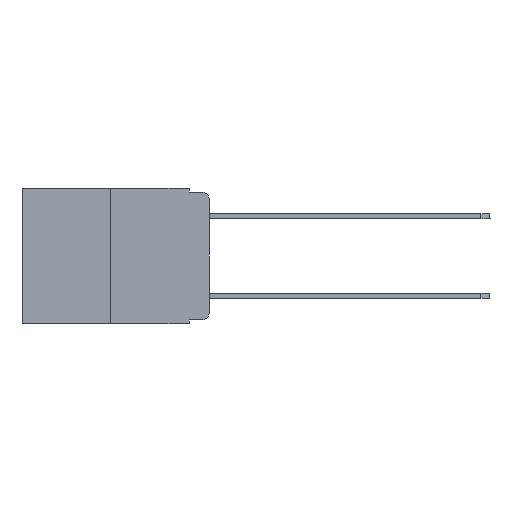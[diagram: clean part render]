
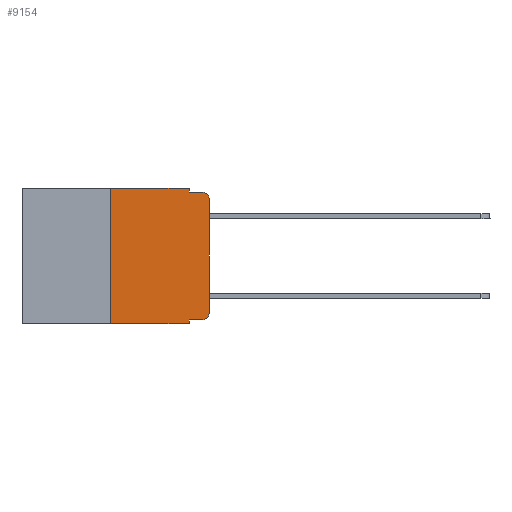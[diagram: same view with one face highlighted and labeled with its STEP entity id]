
A CAD part, left-side view. The second image highlights one B-rep face of the part: STEP entity #9154.
In plain terms, the highlighted planar face has unit normal (-1, 0, 0).
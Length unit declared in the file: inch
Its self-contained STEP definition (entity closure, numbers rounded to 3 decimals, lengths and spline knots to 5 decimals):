
#25 = VERTEX_POINT ( 'NONE', #19356 ) ;
#434 = LINE ( 'NONE', #15198, #15115 ) ;
#866 = EDGE_CURVE ( 'NONE', #24157, #17424, #7147, .T. ) ;
#1061 = VERTEX_POINT ( 'NONE', #18509 ) ;
#1242 = CARTESIAN_POINT ( 'NONE',  ( 0., 0.02, -0.01 ) ) ;
#1291 = VERTEX_POINT ( 'NONE', #17629 ) ;
#1494 = VECTOR ( 'NONE', #23432, 39.37008 ) ;
#1907 = CARTESIAN_POINT ( 'NONE',  ( 0., 0.473, 0. ) ) ;
#2144 = LINE ( 'NONE', #1907, #1494 ) ;
#2804 = AXIS2_PLACEMENT_3D ( 'NONE', #24167, #12146, #20077 ) ;
#2865 = EDGE_LOOP ( 'NONE', ( #8714, #7550, #20555, #15743, #14621, #13286, #20670, #7445, #11721, #8151 ) ) ;
#4114 = AXIS2_PLACEMENT_3D ( 'NONE', #14747, #18538, #8927 ) ;
#5445 = CIRCLE ( 'NONE', #11954, 0.02 ) ;
#5854 = VECTOR ( 'NONE', #7335, 39.37008 ) ;
#7005 = PLANE ( 'NONE',  #4114 ) ;
#7147 = LINE ( 'NONE', #18247, #18322 ) ;
#7335 = DIRECTION ( 'NONE',  ( 0., -1., 0. ) ) ;
#7445 = ORIENTED_EDGE ( 'NONE', *, *, #866, .F. ) ;
#7550 = ORIENTED_EDGE ( 'NONE', *, *, #15150, .T. ) ;
#8151 = ORIENTED_EDGE ( 'NONE', *, *, #22663, .T. ) ;
#8714 = ORIENTED_EDGE ( 'NONE', *, *, #22346, .T. ) ;
#8927 = DIRECTION ( 'NONE',  ( 0., 0., -1. ) ) ;
#9154 = ADVANCED_FACE ( 'NONE', ( #22517 ), #7005, .F. ) ;
#9175 = CARTESIAN_POINT ( 'NONE',  ( 0., 0.051, 0. ) ) ;
#10371 = DIRECTION ( 'NONE',  ( 0., 0., -1. ) ) ;
#10519 = DIRECTION ( 'NONE',  ( 0., -1., 0. ) ) ;
#11162 = VERTEX_POINT ( 'NONE', #25620 ) ;
#11721 = ORIENTED_EDGE ( 'NONE', *, *, #12406, .T. ) ;
#11954 = AXIS2_PLACEMENT_3D ( 'NONE', #12376, #16389, #20480 ) ;
#12146 = DIRECTION ( 'NONE',  ( -1., 0., 0. ) ) ;
#12274 = EDGE_CURVE ( 'NONE', #17093, #19884, #12363, .T. ) ;
#12363 = LINE ( 'NONE', #9175, #15525 ) ;
#12376 = CARTESIAN_POINT ( 'NONE',  ( 0., 0.02, -0.313 ) ) ;
#12406 = EDGE_CURVE ( 'NONE', #24157, #1291, #21729, .T. ) ;
#12481 = DIRECTION ( 'NONE',  ( 0., 0., 1. ) ) ;
#12489 = VECTOR ( 'NONE', #10519, 39.37008 ) ;
#13286 = ORIENTED_EDGE ( 'NONE', *, *, #13308, .F. ) ;
#13308 = EDGE_CURVE ( 'NONE', #20504, #1061, #24518, .T. ) ;
#14159 = CARTESIAN_POINT ( 'NONE',  ( 0., 0.25, -0.343 ) ) ;
#14178 = VECTOR ( 'NONE', #17521, 39.37008 ) ;
#14415 = CARTESIAN_POINT ( 'NONE',  ( 0., 0.25, 0. ) ) ;
#14621 = ORIENTED_EDGE ( 'NONE', *, *, #19229, .F. ) ;
#14747 = CARTESIAN_POINT ( 'NONE',  ( 0., 0.473, 0. ) ) ;
#15115 = VECTOR ( 'NONE', #25752, 39.37008 ) ;
#15150 = EDGE_CURVE ( 'NONE', #11162, #17390, #25397, .T. ) ;
#15198 = CARTESIAN_POINT ( 'NONE',  ( 0., 0., 0. ) ) ;
#15525 = VECTOR ( 'NONE', #18880, 39.37008 ) ;
#15743 = ORIENTED_EDGE ( 'NONE', *, *, #12274, .F. ) ;
#15857 = CARTESIAN_POINT ( 'NONE',  ( 0., 0.051, -0.01 ) ) ;
#16389 = DIRECTION ( 'NONE',  ( -1., 0., 0. ) ) ;
#17093 = VERTEX_POINT ( 'NONE', #19500 ) ;
#17114 = CARTESIAN_POINT ( 'NONE',  ( 0., 0.051, -0.01 ) ) ;
#17390 = VERTEX_POINT ( 'NONE', #1242 ) ;
#17424 = VERTEX_POINT ( 'NONE', #22532 ) ;
#17488 = EDGE_CURVE ( 'NONE', #19884, #17390, #23083, .T. ) ;
#17521 = DIRECTION ( 'NONE',  ( 0., -1., 0. ) ) ;
#17629 = CARTESIAN_POINT ( 'NONE',  ( 0., 0.02, -0.333 ) ) ;
#17922 = CARTESIAN_POINT ( 'NONE',  ( 0., 0.051, -0.333 ) ) ;
#18247 = CARTESIAN_POINT ( 'NONE',  ( 0., 0.051, 0. ) ) ;
#18322 = VECTOR ( 'NONE', #10371, 39.37008 ) ;
#18509 = CARTESIAN_POINT ( 'NONE',  ( 0., 0.25, 0. ) ) ;
#18538 = DIRECTION ( 'NONE',  ( 1., 0., 0. ) ) ;
#18880 = DIRECTION ( 'NONE',  ( 0., 0., -1. ) ) ;
#19229 = EDGE_CURVE ( 'NONE', #1061, #17093, #2144, .T. ) ;
#19356 = CARTESIAN_POINT ( 'NONE',  ( 0., 0., -0.313 ) ) ;
#19500 = CARTESIAN_POINT ( 'NONE',  ( 0., 0.051, 0. ) ) ;
#19540 = CARTESIAN_POINT ( 'NONE',  ( 0., 0.473, -0.343 ) ) ;
#19884 = VERTEX_POINT ( 'NONE', #15857 ) ;
#20077 = DIRECTION ( 'NONE',  ( 0., 0., -1. ) ) ;
#20480 = DIRECTION ( 'NONE',  ( 0., 0., -1. ) ) ;
#20504 = VERTEX_POINT ( 'NONE', #14159 ) ;
#20555 = ORIENTED_EDGE ( 'NONE', *, *, #17488, .F. ) ;
#20670 = ORIENTED_EDGE ( 'NONE', *, *, #22453, .T. ) ;
#21709 = VECTOR ( 'NONE', #12481, 39.37008 ) ;
#21729 = LINE ( 'NONE', #23070, #5854 ) ;
#22346 = EDGE_CURVE ( 'NONE', #25, #11162, #434, .T. ) ;
#22453 = EDGE_CURVE ( 'NONE', #20504, #17424, #22581, .T. ) ;
#22517 = FACE_OUTER_BOUND ( 'NONE', #2865, .T. ) ;
#22532 = CARTESIAN_POINT ( 'NONE',  ( 0., 0.051, -0.343 ) ) ;
#22581 = LINE ( 'NONE', #19540, #14178 ) ;
#22663 = EDGE_CURVE ( 'NONE', #1291, #25, #5445, .T. ) ;
#23070 = CARTESIAN_POINT ( 'NONE',  ( 0., 0.051, -0.333 ) ) ;
#23083 = LINE ( 'NONE', #17114, #12489 ) ;
#23432 = DIRECTION ( 'NONE',  ( 0., -1., 0. ) ) ;
#24157 = VERTEX_POINT ( 'NONE', #17922 ) ;
#24167 = CARTESIAN_POINT ( 'NONE',  ( 0., 0.02, -0.03 ) ) ;
#24518 = LINE ( 'NONE', #14415, #21709 ) ;
#25397 = CIRCLE ( 'NONE', #2804, 0.02 ) ;
#25620 = CARTESIAN_POINT ( 'NONE',  ( 0., 0., -0.03 ) ) ;
#25752 = DIRECTION ( 'NONE',  ( 0., 0., 1. ) ) ;
